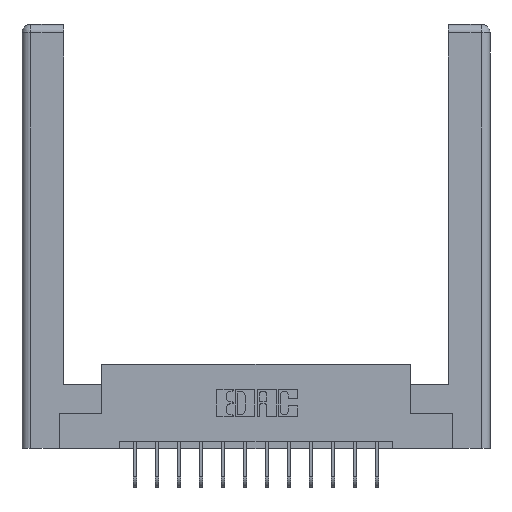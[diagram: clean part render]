
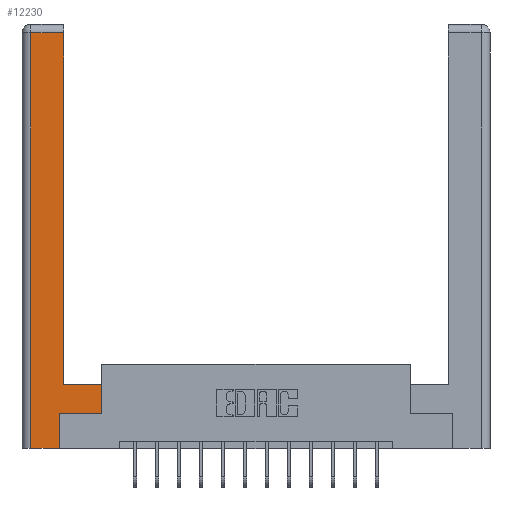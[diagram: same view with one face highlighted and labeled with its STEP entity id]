
A CAD part, top view. The second image highlights one B-rep face of the part: STEP entity #12230.
In plain terms, the highlighted planar face has unit normal (0, 0, 1).
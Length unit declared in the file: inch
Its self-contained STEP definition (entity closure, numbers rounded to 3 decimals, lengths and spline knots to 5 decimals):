
#489 = CARTESIAN_POINT ( 'NONE',  ( 0.0615, 2.94, 0. ) ) ;
#773 = CARTESIAN_POINT ( 'NONE',  ( 0., 0., 0. ) ) ;
#1083 = DIRECTION ( 'NONE',  ( 1., 0., 0. ) ) ;
#1192 = CARTESIAN_POINT ( 'NONE',  ( 0.565, 0.245, 0. ) ) ;
#1601 = VERTEX_POINT ( 'NONE', #6656 ) ;
#2261 = ORIENTED_EDGE ( 'NONE', *, *, #12999, .T. ) ;
#3198 = LINE ( 'NONE', #14324, #13043 ) ;
#3610 = CARTESIAN_POINT ( 'NONE',  ( 0.265, 0.245, 0. ) ) ;
#4294 = VECTOR ( 'NONE', #12358, 39.37008 ) ;
#4341 = CARTESIAN_POINT ( 'NONE',  ( 0.0615, 2.94, 0. ) ) ;
#4698 = CARTESIAN_POINT ( 'NONE',  ( 0.265, 0.245, 0. ) ) ;
#4829 = ORIENTED_EDGE ( 'NONE', *, *, #15490, .T. ) ;
#5413 = LINE ( 'NONE', #5554, #12718 ) ;
#5554 = CARTESIAN_POINT ( 'NONE',  ( 0.265, 0., 0. ) ) ;
#5874 = EDGE_CURVE ( 'NONE', #15931, #7560, #8683, .T. ) ;
#6297 = DIRECTION ( 'NONE',  ( 1., 0., 0. ) ) ;
#6656 = CARTESIAN_POINT ( 'NONE',  ( 0.565, 0.45, 0. ) ) ;
#6750 = DIRECTION ( 'NONE',  ( 0., -1., 0. ) ) ;
#6884 = CARTESIAN_POINT ( 'NONE',  ( 0.0615, 0., 0. ) ) ;
#7313 = FACE_OUTER_BOUND ( 'NONE', #13556, .T. ) ;
#7421 = CARTESIAN_POINT ( 'NONE',  ( 0.0615, 0., 0. ) ) ;
#7560 = VERTEX_POINT ( 'NONE', #3610 ) ;
#7851 = VERTEX_POINT ( 'NONE', #4341 ) ;
#7987 = LINE ( 'NONE', #489, #16301 ) ;
#8063 = CARTESIAN_POINT ( 'NONE',  ( 0.295, 0.45, 0. ) ) ;
#8683 = LINE ( 'NONE', #4698, #12286 ) ;
#8832 = DIRECTION ( 'NONE',  ( -1., 0., 0. ) ) ;
#8950 = DIRECTION ( 'NONE',  ( 0., 1., 0. ) ) ;
#9111 = CARTESIAN_POINT ( 'NONE',  ( 0.295, 2.94, 0. ) ) ;
#9498 = CARTESIAN_POINT ( 'NONE',  ( 0.565, 0.245, 0. ) ) ;
#9537 = EDGE_CURVE ( 'NONE', #7560, #15424, #12508, .T. ) ;
#9917 = EDGE_CURVE ( 'NONE', #13432, #15931, #5413, .T. ) ;
#10031 = DIRECTION ( 'NONE',  ( -1., 0., 0. ) ) ;
#10306 = DIRECTION ( 'NONE',  ( 0., 1., 0. ) ) ;
#10365 = ORIENTED_EDGE ( 'NONE', *, *, #11078, .T. ) ;
#10460 = VERTEX_POINT ( 'NONE', #17533 ) ;
#11078 = EDGE_CURVE ( 'NONE', #14494, #7851, #7987, .T. ) ;
#11162 = ORIENTED_EDGE ( 'NONE', *, *, #9537, .T. ) ;
#11455 = ORIENTED_EDGE ( 'NONE', *, *, #9917, .T. ) ;
#11696 = ORIENTED_EDGE ( 'NONE', *, *, #13158, .T. ) ;
#12230 = ADVANCED_FACE ( 'NONE', ( #7313 ), #15722, .F. ) ;
#12241 = ORIENTED_EDGE ( 'NONE', *, *, #16455, .T. ) ;
#12286 = VECTOR ( 'NONE', #10306, 39.37008 ) ;
#12358 = DIRECTION ( 'NONE',  ( 0., 1., 0. ) ) ;
#12508 = LINE ( 'NONE', #1192, #16560 ) ;
#12702 = CARTESIAN_POINT ( 'NONE',  ( 0.265, 0., 0. ) ) ;
#12718 = VECTOR ( 'NONE', #6297, 39.37008 ) ;
#12999 = EDGE_CURVE ( 'NONE', #10460, #14494, #3198, .T. ) ;
#13043 = VECTOR ( 'NONE', #8950, 39.37008 ) ;
#13048 = AXIS2_PLACEMENT_3D ( 'NONE', #773, #16985, #8832 ) ;
#13158 = EDGE_CURVE ( 'NONE', #7851, #13432, #13660, .T. ) ;
#13432 = VERTEX_POINT ( 'NONE', #7421 ) ;
#13556 = EDGE_LOOP ( 'NONE', ( #2261, #10365, #11696, #11455, #13996, #11162, #4829, #12241 ) ) ;
#13660 = LINE ( 'NONE', #6884, #14947 ) ;
#13914 = VECTOR ( 'NONE', #17448, 39.37008 ) ;
#13996 = ORIENTED_EDGE ( 'NONE', *, *, #5874, .T. ) ;
#14324 = CARTESIAN_POINT ( 'NONE',  ( 0.295, 3., 0. ) ) ;
#14494 = VERTEX_POINT ( 'NONE', #9111 ) ;
#14947 = VECTOR ( 'NONE', #6750, 39.37008 ) ;
#15237 = LINE ( 'NONE', #16475, #4294 ) ;
#15424 = VERTEX_POINT ( 'NONE', #9498 ) ;
#15490 = EDGE_CURVE ( 'NONE', #15424, #1601, #15237, .T. ) ;
#15722 = PLANE ( 'NONE',  #13048 ) ;
#15931 = VERTEX_POINT ( 'NONE', #12702 ) ;
#16301 = VECTOR ( 'NONE', #10031, 39.37008 ) ;
#16455 = EDGE_CURVE ( 'NONE', #1601, #10460, #17500, .T. ) ;
#16475 = CARTESIAN_POINT ( 'NONE',  ( 0.565, 0.45, 0. ) ) ;
#16560 = VECTOR ( 'NONE', #1083, 39.37008 ) ;
#16985 = DIRECTION ( 'NONE',  ( 0., 0., -1. ) ) ;
#17448 = DIRECTION ( 'NONE',  ( -1., 0., 0. ) ) ;
#17500 = LINE ( 'NONE', #8063, #13914 ) ;
#17533 = CARTESIAN_POINT ( 'NONE',  ( 0.295, 0.45, 0. ) ) ;
